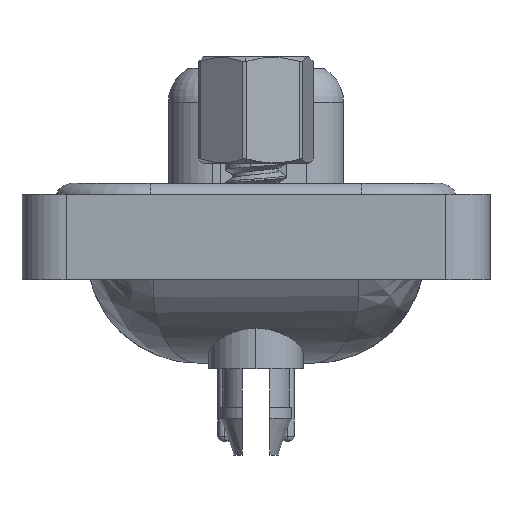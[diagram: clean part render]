
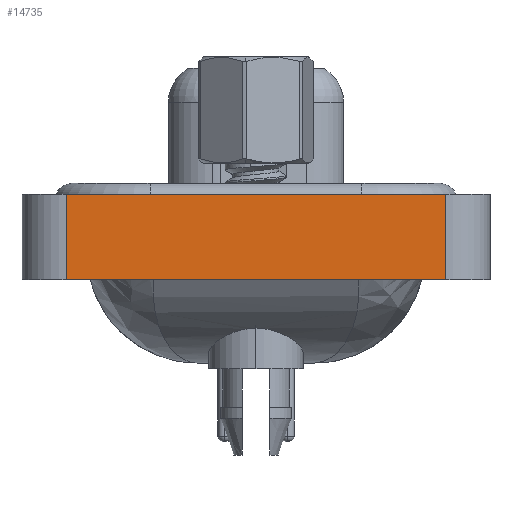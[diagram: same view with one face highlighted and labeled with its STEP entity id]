
A CAD part, left-side view. The second image highlights one B-rep face of the part: STEP entity #14735.
In plain terms, the highlighted planar face has unit normal (-1, 0, 0).
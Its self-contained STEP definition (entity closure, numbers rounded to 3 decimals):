
#429 = VECTOR ( 'NONE', #11468, 1000. ) ;
#486 = CARTESIAN_POINT ( 'NONE',  ( -7.35, 8.55, -3.35 ) ) ;
#1875 = VERTEX_POINT ( 'NONE', #17197 ) ;
#2100 = CARTESIAN_POINT ( 'NONE',  ( -7.35, -8.55, -3.35 ) ) ;
#3040 = PLANE ( 'NONE',  #5407 ) ;
#3713 = CARTESIAN_POINT ( 'NONE',  ( -7.35, 8.55, 0.5 ) ) ;
#4846 = LINE ( 'NONE', #14197, #21805 ) ;
#5407 = AXIS2_PLACEMENT_3D ( 'NONE', #12764, #6952, #20731 ) ;
#6000 = CARTESIAN_POINT ( 'NONE',  ( -7.35, -8.55, 0.5 ) ) ;
#6128 = EDGE_CURVE ( 'NONE', #1875, #6988, #4846, .T. ) ;
#6154 = DIRECTION ( 'NONE',  ( 0., 0., 1. ) ) ;
#6952 = DIRECTION ( 'NONE',  ( -1., 0., 0. ) ) ;
#6988 = VERTEX_POINT ( 'NONE', #6000 ) ;
#7621 = CARTESIAN_POINT ( 'NONE',  ( -7.35, -8.55, 0.5 ) ) ;
#8391 = DIRECTION ( 'NONE',  ( 0., 0., 1. ) ) ;
#8688 = VERTEX_POINT ( 'NONE', #24608 ) ;
#10281 = EDGE_CURVE ( 'NONE', #23045, #6988, #21159, .T. ) ;
#11468 = DIRECTION ( 'NONE',  ( 0., -1., 0. ) ) ;
#11899 = EDGE_CURVE ( 'NONE', #8688, #1875, #21561, .T. ) ;
#12764 = CARTESIAN_POINT ( 'NONE',  ( -7.35, -8.55, -3.35 ) ) ;
#12840 = VECTOR ( 'NONE', #6154, 1000. ) ;
#13296 = ORIENTED_EDGE ( 'NONE', *, *, #24063, .F. ) ;
#14197 = CARTESIAN_POINT ( 'NONE',  ( -7.35, -8.55, -3.35 ) ) ;
#14735 = ADVANCED_FACE ( 'NONE', ( #18709 ), #3040, .T. ) ;
#15460 = DIRECTION ( 'NONE',  ( 0., -1., 0. ) ) ;
#16712 = ORIENTED_EDGE ( 'NONE', *, *, #10281, .F. ) ;
#17197 = CARTESIAN_POINT ( 'NONE',  ( -7.35, -8.55, -3.35 ) ) ;
#17787 = EDGE_LOOP ( 'NONE', ( #19631, #16712, #13296, #21198 ) ) ;
#18709 = FACE_OUTER_BOUND ( 'NONE', #17787, .T. ) ;
#19631 = ORIENTED_EDGE ( 'NONE', *, *, #6128, .T. ) ;
#20731 = DIRECTION ( 'NONE',  ( 0., 0., 1. ) ) ;
#21159 = LINE ( 'NONE', #7621, #22957 ) ;
#21198 = ORIENTED_EDGE ( 'NONE', *, *, #11899, .T. ) ;
#21561 = LINE ( 'NONE', #2100, #429 ) ;
#21805 = VECTOR ( 'NONE', #8391, 1000. ) ;
#22957 = VECTOR ( 'NONE', #15460, 1000. ) ;
#23045 = VERTEX_POINT ( 'NONE', #3713 ) ;
#23493 = LINE ( 'NONE', #486, #12840 ) ;
#24063 = EDGE_CURVE ( 'NONE', #8688, #23045, #23493, .T. ) ;
#24608 = CARTESIAN_POINT ( 'NONE',  ( -7.35, 8.55, -3.35 ) ) ;
